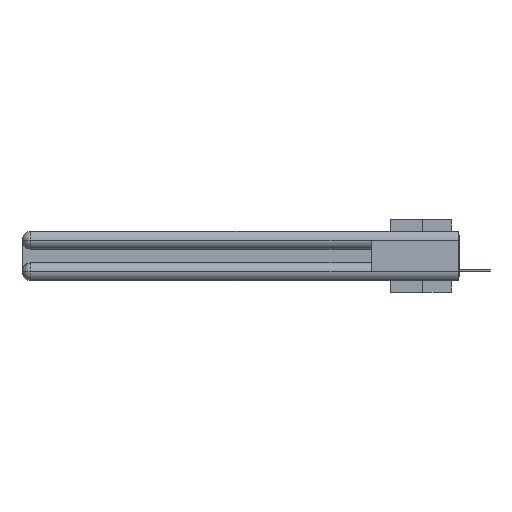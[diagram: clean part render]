
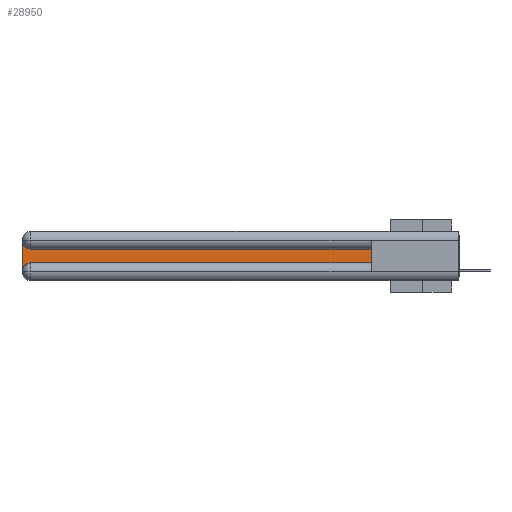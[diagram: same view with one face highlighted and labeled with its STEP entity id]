
A CAD part, left-side view. The second image highlights one B-rep face of the part: STEP entity #28950.
In plain terms, the highlighted planar face has unit normal (-1, 0, 0).
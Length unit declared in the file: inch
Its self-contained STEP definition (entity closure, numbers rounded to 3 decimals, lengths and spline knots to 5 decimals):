
#370 = DIRECTION ( 'NONE',  ( 0., 0., -1. ) ) ;
#1073 = VERTEX_POINT ( 'NONE', #26487 ) ;
#2096 = ORIENTED_EDGE ( 'NONE', *, *, #29936, .T. ) ;
#2645 = LINE ( 'NONE', #24154, #27978 ) ;
#3169 = CARTESIAN_POINT ( 'NONE',  ( 0.075, 2.94, -0.2775 ) ) ;
#4070 = DIRECTION ( 'NONE',  ( 1., 0., 0. ) ) ;
#4271 = CARTESIAN_POINT ( 'NONE',  ( 0.075, 2.94, -0.0625 ) ) ;
#4393 = CARTESIAN_POINT ( 'NONE',  ( 0.075, 2.94, -0.2175 ) ) ;
#4506 = EDGE_LOOP ( 'NONE', ( #2096, #32548, #14118, #35755, #31951, #7979 ) ) ;
#4821 = VECTOR ( 'NONE', #18714, 39.37008 ) ;
#7548 = AXIS2_PLACEMENT_3D ( 'NONE', #3169, #33050, #370 ) ;
#7979 = ORIENTED_EDGE ( 'NONE', *, *, #25085, .T. ) ;
#8469 = VERTEX_POINT ( 'NONE', #36483 ) ;
#9457 = FACE_OUTER_BOUND ( 'NONE', #4506, .T. ) ;
#9528 = EDGE_CURVE ( 'NONE', #18285, #1073, #15824, .T. ) ;
#10027 = CARTESIAN_POINT ( 'NONE',  ( 0.075, 3., -0.1225 ) ) ;
#10743 = VERTEX_POINT ( 'NONE', #19431 ) ;
#10953 = CARTESIAN_POINT ( 'NONE',  ( 0.075, 0.6, -0.2175 ) ) ;
#11625 = VERTEX_POINT ( 'NONE', #10953 ) ;
#12192 = EDGE_CURVE ( 'NONE', #1073, #10743, #31237, .T. ) ;
#12319 = VECTOR ( 'NONE', #20226, 39.37008 ) ;
#14118 = ORIENTED_EDGE ( 'NONE', *, *, #12192, .T. ) ;
#15824 = CIRCLE ( 'NONE', #20248, 0.06 ) ;
#15827 = DIRECTION ( 'NONE',  ( 1., 0., 0. ) ) ;
#17742 = LINE ( 'NONE', #36028, #19376 ) ;
#18133 = DIRECTION ( 'NONE',  ( 0., -1., 0. ) ) ;
#18285 = VERTEX_POINT ( 'NONE', #26139 ) ;
#18714 = DIRECTION ( 'NONE',  ( 0., 0., -1. ) ) ;
#19376 = VECTOR ( 'NONE', #18133, 39.37008 ) ;
#19431 = CARTESIAN_POINT ( 'NONE',  ( 0.075, 3., -0.2775 ) ) ;
#20226 = DIRECTION ( 'NONE',  ( 0., 1., 0. ) ) ;
#20248 = AXIS2_PLACEMENT_3D ( 'NONE', #4271, #4070, #28738 ) ;
#20404 = CARTESIAN_POINT ( 'NONE',  ( 0.075, 0.6, -0.1225 ) ) ;
#21489 = CARTESIAN_POINT ( 'NONE',  ( 0.075, 3., -0.2175 ) ) ;
#22167 = DIRECTION ( 'NONE',  ( 0., 0., -1. ) ) ;
#23390 = LINE ( 'NONE', #20404, #12319 ) ;
#24154 = CARTESIAN_POINT ( 'NONE',  ( 0.075, 0.6, -0.2175 ) ) ;
#25085 = EDGE_CURVE ( 'NONE', #11625, #8469, #2645, .T. ) ;
#25868 = CIRCLE ( 'NONE', #7548, 0.06 ) ;
#26139 = CARTESIAN_POINT ( 'NONE',  ( 0.075, 2.94, -0.1225 ) ) ;
#26487 = CARTESIAN_POINT ( 'NONE',  ( 0.075, 3., -0.0625 ) ) ;
#27978 = VECTOR ( 'NONE', #33122, 39.37008 ) ;
#28738 = DIRECTION ( 'NONE',  ( 0., 0., -1. ) ) ;
#28950 = ADVANCED_FACE ( 'NONE', ( #9457 ), #37477, .F. ) ;
#29936 = EDGE_CURVE ( 'NONE', #8469, #18285, #23390, .T. ) ;
#30162 = AXIS2_PLACEMENT_3D ( 'NONE', #10027, #15827, #22167 ) ;
#30937 = EDGE_CURVE ( 'NONE', #34566, #11625, #17742, .T. ) ;
#31237 = LINE ( 'NONE', #21489, #4821 ) ;
#31951 = ORIENTED_EDGE ( 'NONE', *, *, #30937, .T. ) ;
#32548 = ORIENTED_EDGE ( 'NONE', *, *, #9528, .T. ) ;
#33050 = DIRECTION ( 'NONE',  ( 1., 0., 0. ) ) ;
#33122 = DIRECTION ( 'NONE',  ( 0., 0., 1. ) ) ;
#34566 = VERTEX_POINT ( 'NONE', #4393 ) ;
#34881 = EDGE_CURVE ( 'NONE', #10743, #34566, #25868, .T. ) ;
#35755 = ORIENTED_EDGE ( 'NONE', *, *, #34881, .T. ) ;
#36028 = CARTESIAN_POINT ( 'NONE',  ( 0.075, 0.6, -0.2175 ) ) ;
#36483 = CARTESIAN_POINT ( 'NONE',  ( 0.075, 0.6, -0.1225 ) ) ;
#37477 = PLANE ( 'NONE',  #30162 ) ;
